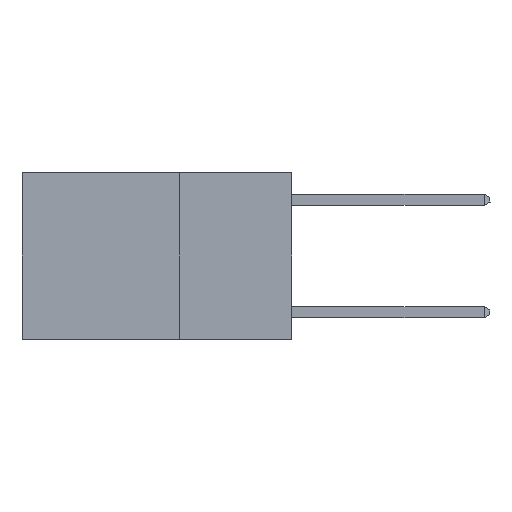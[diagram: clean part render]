
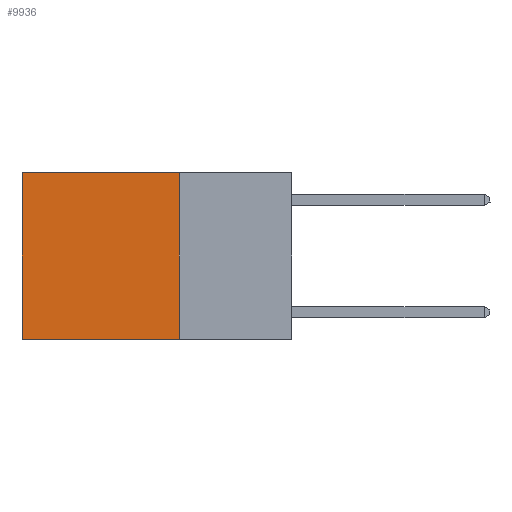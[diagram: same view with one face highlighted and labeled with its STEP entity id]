
A CAD part, left-side view. The second image highlights one B-rep face of the part: STEP entity #9936.
In plain terms, the highlighted planar face has unit normal (-1, 0, 0).
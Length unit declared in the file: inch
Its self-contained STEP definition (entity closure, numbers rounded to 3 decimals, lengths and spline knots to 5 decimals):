
#180 = VERTEX_POINT ( 'NONE', #27707 ) ;
#1054 = LINE ( 'NONE', #14732, #15216 ) ;
#1377 = DIRECTION ( 'NONE',  ( 1., 0., 0. ) ) ;
#5793 = DIRECTION ( 'NONE',  ( 0., 0., -1. ) ) ;
#7549 = VECTOR ( 'NONE', #7922, 39.37008 ) ;
#7574 = AXIS2_PLACEMENT_3D ( 'NONE', #14565, #1377, #10252 ) ;
#7922 = DIRECTION ( 'NONE',  ( 0., 1., 0. ) ) ;
#8752 = EDGE_LOOP ( 'NONE', ( #24653, #18352, #9055, #10399 ) ) ;
#9055 = ORIENTED_EDGE ( 'NONE', *, *, #9685, .F. ) ;
#9271 = DIRECTION ( 'NONE',  ( 0., 1., 0. ) ) ;
#9685 = EDGE_CURVE ( 'NONE', #17018, #21052, #19695, .T. ) ;
#9690 = CARTESIAN_POINT ( 'NONE',  ( 0.2625, 0.25, 0. ) ) ;
#9936 = ADVANCED_FACE ( 'NONE', ( #27575 ), #25569, .F. ) ;
#9947 = VERTEX_POINT ( 'NONE', #14470 ) ;
#10252 = DIRECTION ( 'NONE',  ( 0., 0., -1. ) ) ;
#10399 = ORIENTED_EDGE ( 'NONE', *, *, #19555, .T. ) ;
#12261 = CARTESIAN_POINT ( 'NONE',  ( 0.2625, 0.25, 0. ) ) ;
#14470 = CARTESIAN_POINT ( 'NONE',  ( 0.2625, 0.6, -0.37 ) ) ;
#14565 = CARTESIAN_POINT ( 'NONE',  ( 0.2625, 0.25, 0. ) ) ;
#14732 = CARTESIAN_POINT ( 'NONE',  ( 0.2625, 0.6, 0. ) ) ;
#15216 = VECTOR ( 'NONE', #5793, 39.37008 ) ;
#17018 = VERTEX_POINT ( 'NONE', #9690 ) ;
#17747 = CARTESIAN_POINT ( 'NONE',  ( 0.2625, 0.25, -0.37 ) ) ;
#18312 = VECTOR ( 'NONE', #23921, 39.37008 ) ;
#18352 = ORIENTED_EDGE ( 'NONE', *, *, #24874, .F. ) ;
#18396 = EDGE_CURVE ( 'NONE', #180, #9947, #1054, .T. ) ;
#18579 = LINE ( 'NONE', #12261, #7549 ) ;
#19555 = EDGE_CURVE ( 'NONE', #17018, #180, #18579, .T. ) ;
#19695 = LINE ( 'NONE', #21427, #18312 ) ;
#19947 = CARTESIAN_POINT ( 'NONE',  ( 0.2625, 0.25, -0.37 ) ) ;
#21052 = VERTEX_POINT ( 'NONE', #17747 ) ;
#21427 = CARTESIAN_POINT ( 'NONE',  ( 0.2625, 0.25, 0. ) ) ;
#23921 = DIRECTION ( 'NONE',  ( 0., 0., -1. ) ) ;
#24653 = ORIENTED_EDGE ( 'NONE', *, *, #18396, .T. ) ;
#24863 = LINE ( 'NONE', #19947, #25197 ) ;
#24874 = EDGE_CURVE ( 'NONE', #21052, #9947, #24863, .T. ) ;
#25197 = VECTOR ( 'NONE', #9271, 39.37008 ) ;
#25569 = PLANE ( 'NONE',  #7574 ) ;
#27575 = FACE_OUTER_BOUND ( 'NONE', #8752, .T. ) ;
#27707 = CARTESIAN_POINT ( 'NONE',  ( 0.2625, 0.6, 0. ) ) ;
